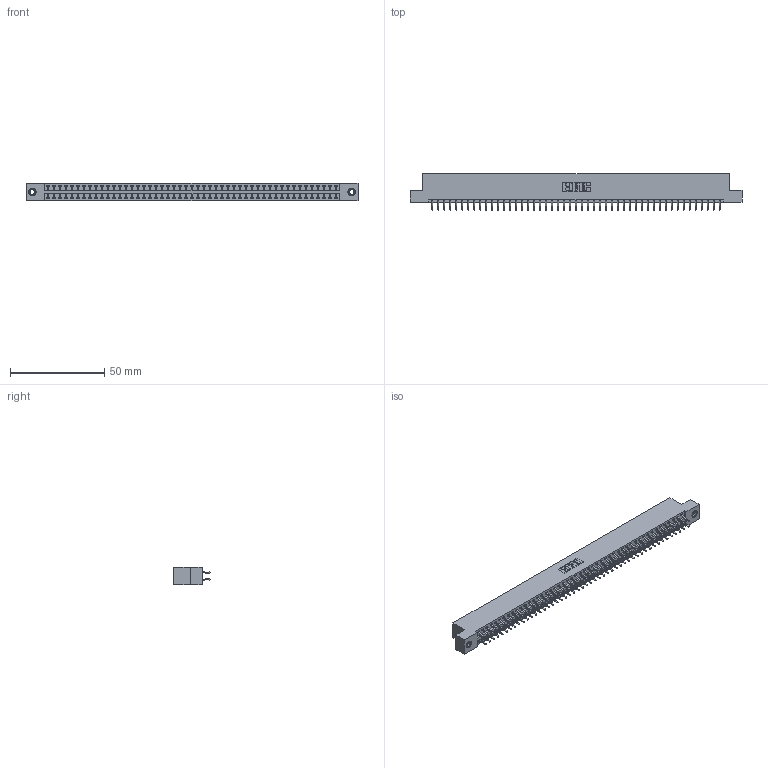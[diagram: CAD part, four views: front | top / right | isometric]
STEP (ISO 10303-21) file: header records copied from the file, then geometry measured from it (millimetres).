
FILE_DESCRIPTION (( 'STEP AP203' ), '1' );
FILE_NAME ('396-098-556-207.STEP', '2018-09-14T05:37:13', ( '' ), ( '' ), 'SwSTEP 2.0', 'SolidWorks 2016', '' );
FILE_SCHEMA (( 'CONFIG_CONTROL_DESIGN' ));
Length unit declared in the file: inch
Products named in the file (4): 396-098-556-207; 346 Part_Flush Mounting Lugs - 0.156 Dia-TI; 345-292-001_556 Tail; 345-250-001_345-250-005-103
Assembly tree (101 placements, depth 2):
  396-098-556-207
    346 Part_Flush Mounting Lugs - 0.156 Dia-TI
    345-292-001_556 Tail  x98
    345-250-001_345-250-005-103  x2
Bounding box: 176.15 x 19.57 x 9.4 mm (x, y, z)
Volume: 17213.7 mm3; surface area: 23714.1 mm2
Topology: 101 solids, 101 shells, 5866 faces, 17419 edges, 11474 vertices
Faces by surface type: plane 3930, cylinder 1920, cone 12, torus 4
Entity records: 32442 total; most frequent: CARTESIAN_POINT 5335, ORIENTED_EDGE 5250, DIRECTION 4767, EDGE_CURVE 2625, LINE 2269, VECTOR 2269, VERTEX_POINT 1744, AXIS2_PLACEMENT_3D 1249
